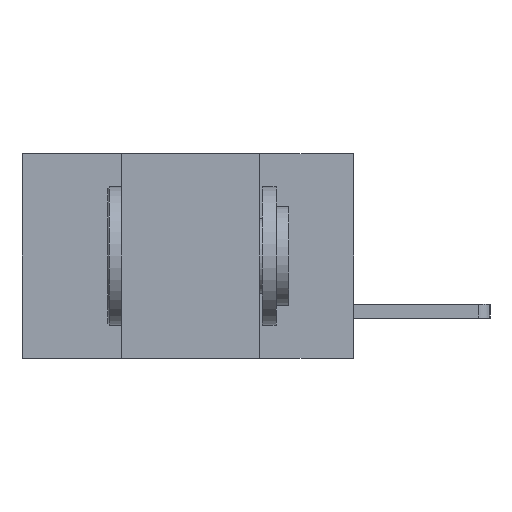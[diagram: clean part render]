
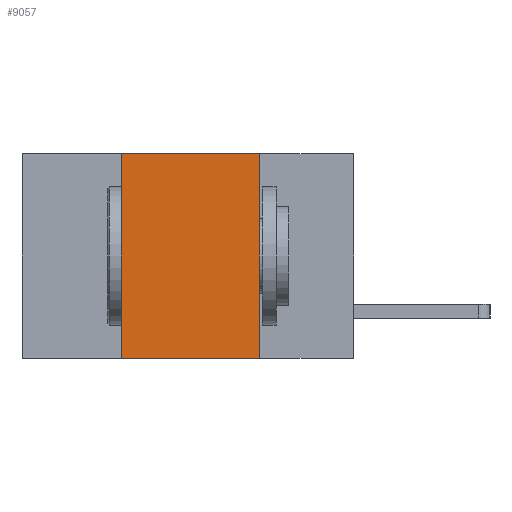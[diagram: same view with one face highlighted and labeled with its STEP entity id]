
A CAD part, left-side view. The second image highlights one B-rep face of the part: STEP entity #9057.
In plain terms, the highlighted planar face has unit normal (-1, 0, 0).
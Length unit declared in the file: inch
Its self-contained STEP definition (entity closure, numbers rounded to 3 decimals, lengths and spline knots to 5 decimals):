
#87 = DIRECTION ( 'NONE',  ( 1., 0., 0. ) ) ;
#422 = LINE ( 'NONE', #11475, #2029 ) ;
#617 = VECTOR ( 'NONE', #7152, 39.37008 ) ;
#1173 = PLANE ( 'NONE',  #11650 ) ;
#1660 = EDGE_CURVE ( 'NONE', #11139, #3416, #11729, .T. ) ;
#1749 = CARTESIAN_POINT ( 'NONE',  ( 0., 0.17, 0. ) ) ;
#2029 = VECTOR ( 'NONE', #6828, 39.37008 ) ;
#2658 = VECTOR ( 'NONE', #10140, 39.37008 ) ;
#2703 = EDGE_CURVE ( 'NONE', #6239, #9002, #6984, .T. ) ;
#3416 = VERTEX_POINT ( 'NONE', #9367 ) ;
#4224 = CARTESIAN_POINT ( 'NONE',  ( 0., 0.17, 0. ) ) ;
#4690 = ORIENTED_EDGE ( 'NONE', *, *, #9694, .F. ) ;
#4699 = ORIENTED_EDGE ( 'NONE', *, *, #11780, .T. ) ;
#5699 = CARTESIAN_POINT ( 'NONE',  ( 0., 0.6, 0. ) ) ;
#6022 = VECTOR ( 'NONE', #11037, 39.37008 ) ;
#6239 = VERTEX_POINT ( 'NONE', #11945 ) ;
#6306 = ORIENTED_EDGE ( 'NONE', *, *, #2703, .F. ) ;
#6376 = CARTESIAN_POINT ( 'NONE',  ( 0., 0.6, -0.37 ) ) ;
#6828 = DIRECTION ( 'NONE',  ( 0., -1., 0. ) ) ;
#6984 = LINE ( 'NONE', #10799, #6022 ) ;
#7152 = DIRECTION ( 'NONE',  ( 0., 0., -1. ) ) ;
#7530 = DIRECTION ( 'NONE',  ( 0., 0., -1. ) ) ;
#8365 = FACE_OUTER_BOUND ( 'NONE', #9669, .T. ) ;
#8572 = ORIENTED_EDGE ( 'NONE', *, *, #1660, .F. ) ;
#9002 = VERTEX_POINT ( 'NONE', #9152 ) ;
#9057 = ADVANCED_FACE ( 'NONE', ( #8365 ), #1173, .F. ) ;
#9152 = CARTESIAN_POINT ( 'NONE',  ( 0., 0.42, 0. ) ) ;
#9367 = CARTESIAN_POINT ( 'NONE',  ( 0., 0.17, -0.37 ) ) ;
#9669 = EDGE_LOOP ( 'NONE', ( #8572, #4690, #6306, #4699 ) ) ;
#9694 = EDGE_CURVE ( 'NONE', #9002, #11139, #422, .T. ) ;
#10140 = DIRECTION ( 'NONE',  ( 0., -1., 0. ) ) ;
#10799 = CARTESIAN_POINT ( 'NONE',  ( 0., 0.42, 0. ) ) ;
#11037 = DIRECTION ( 'NONE',  ( 0., 0., 1. ) ) ;
#11139 = VERTEX_POINT ( 'NONE', #1749 ) ;
#11164 = LINE ( 'NONE', #6376, #2658 ) ;
#11475 = CARTESIAN_POINT ( 'NONE',  ( 0., 0.6, 0. ) ) ;
#11650 = AXIS2_PLACEMENT_3D ( 'NONE', #5699, #87, #7530 ) ;
#11729 = LINE ( 'NONE', #4224, #617 ) ;
#11780 = EDGE_CURVE ( 'NONE', #6239, #3416, #11164, .T. ) ;
#11945 = CARTESIAN_POINT ( 'NONE',  ( 0., 0.42, -0.37 ) ) ;
